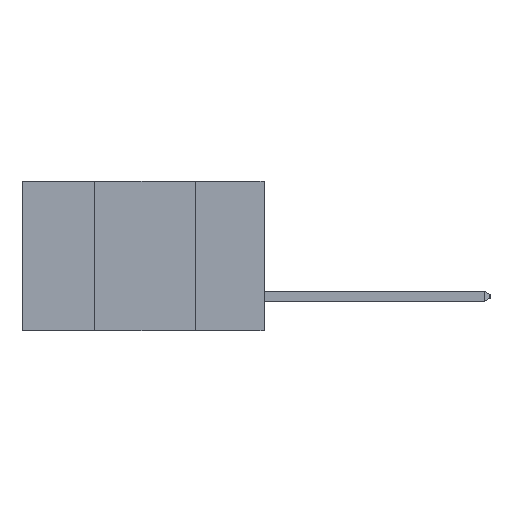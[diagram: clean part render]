
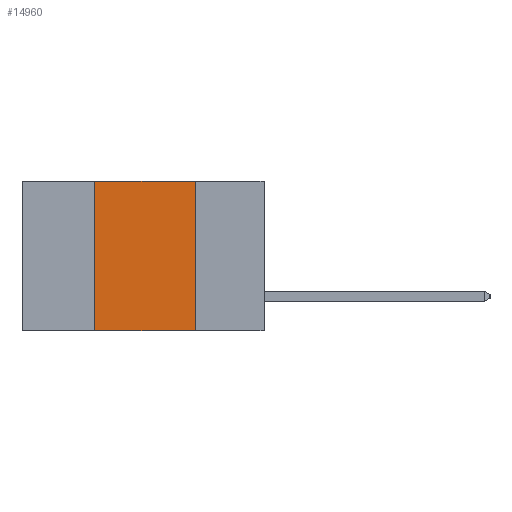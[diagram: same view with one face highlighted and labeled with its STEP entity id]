
A CAD part, left-side view. The second image highlights one B-rep face of the part: STEP entity #14960.
In plain terms, the highlighted planar face has unit normal (-1, 0, 0).
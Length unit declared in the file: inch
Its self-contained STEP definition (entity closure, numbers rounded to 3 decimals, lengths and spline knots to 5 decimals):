
#543 = VECTOR ( 'NONE', #21644, 39.37008 ) ;
#815 = ORIENTED_EDGE ( 'NONE', *, *, #7629, .F. ) ;
#878 = VERTEX_POINT ( 'NONE', #14845 ) ;
#1755 = LINE ( 'NONE', #20535, #20685 ) ;
#2090 = EDGE_CURVE ( 'NONE', #878, #23350, #10543, .T. ) ;
#2140 = DIRECTION ( 'NONE',  ( 0., -1., 0. ) ) ;
#2302 = CARTESIAN_POINT ( 'NONE',  ( 0., 0.6, -0.37 ) ) ;
#3556 = ORIENTED_EDGE ( 'NONE', *, *, #17283, .F. ) ;
#3674 = LINE ( 'NONE', #2302, #8616 ) ;
#5056 = EDGE_CURVE ( 'NONE', #13091, #23350, #3674, .T. ) ;
#6060 = DIRECTION ( 'NONE',  ( 0., 0., 1. ) ) ;
#7381 = ORIENTED_EDGE ( 'NONE', *, *, #2090, .F. ) ;
#7629 = EDGE_CURVE ( 'NONE', #11360, #878, #15449, .T. ) ;
#8616 = VECTOR ( 'NONE', #2140, 39.37008 ) ;
#8873 = CARTESIAN_POINT ( 'NONE',  ( 0., 0.6, 0. ) ) ;
#9706 = FACE_OUTER_BOUND ( 'NONE', #9951, .T. ) ;
#9951 = EDGE_LOOP ( 'NONE', ( #7381, #815, #3556, #17111 ) ) ;
#10543 = LINE ( 'NONE', #12144, #543 ) ;
#10737 = DIRECTION ( 'NONE',  ( 0., 0., -1. ) ) ;
#11360 = VERTEX_POINT ( 'NONE', #17432 ) ;
#12144 = CARTESIAN_POINT ( 'NONE',  ( 0., 0.17, -0.37 ) ) ;
#13091 = VERTEX_POINT ( 'NONE', #19891 ) ;
#14304 = CARTESIAN_POINT ( 'NONE',  ( 0., 0.6, 0. ) ) ;
#14327 = DIRECTION ( 'NONE',  ( 0., -1., 0. ) ) ;
#14845 = CARTESIAN_POINT ( 'NONE',  ( 0., 0.17, 0. ) ) ;
#14960 = ADVANCED_FACE ( 'NONE', ( #9706 ), #19751, .F. ) ;
#15449 = LINE ( 'NONE', #14304, #19605 ) ;
#15874 = CARTESIAN_POINT ( 'NONE',  ( 0., 0.17, -0.37 ) ) ;
#17111 = ORIENTED_EDGE ( 'NONE', *, *, #5056, .T. ) ;
#17283 = EDGE_CURVE ( 'NONE', #13091, #11360, #1755, .T. ) ;
#17432 = CARTESIAN_POINT ( 'NONE',  ( 0., 0.42, 0. ) ) ;
#19605 = VECTOR ( 'NONE', #14327, 39.37008 ) ;
#19751 = PLANE ( 'NONE',  #22730 ) ;
#19891 = CARTESIAN_POINT ( 'NONE',  ( 0., 0.42, -0.37 ) ) ;
#20535 = CARTESIAN_POINT ( 'NONE',  ( 0., 0.42, -0.37 ) ) ;
#20685 = VECTOR ( 'NONE', #6060, 39.37008 ) ;
#21479 = DIRECTION ( 'NONE',  ( 1., 0., 0. ) ) ;
#21644 = DIRECTION ( 'NONE',  ( 0., 0., -1. ) ) ;
#22730 = AXIS2_PLACEMENT_3D ( 'NONE', #8873, #21479, #10737 ) ;
#23350 = VERTEX_POINT ( 'NONE', #15874 ) ;
